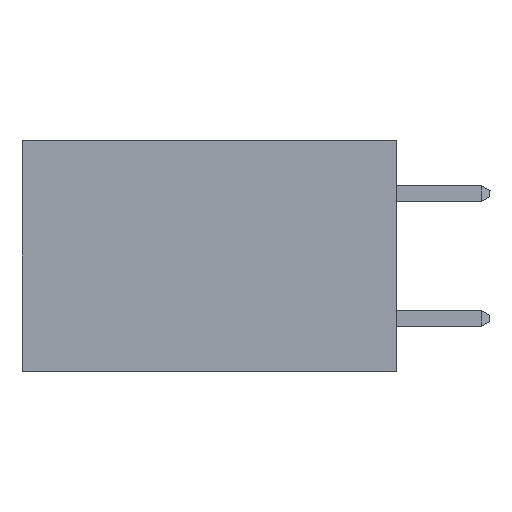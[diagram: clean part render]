
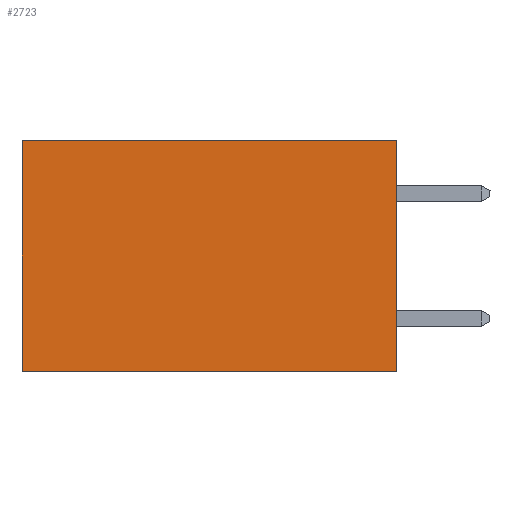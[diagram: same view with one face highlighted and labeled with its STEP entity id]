
A CAD part, left-side view. The second image highlights one B-rep face of the part: STEP entity #2723.
In plain terms, the highlighted planar face has unit normal (-1, 0, 0).
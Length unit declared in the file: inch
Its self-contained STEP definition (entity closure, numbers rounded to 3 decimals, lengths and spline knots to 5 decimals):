
#710 = VERTEX_POINT ( 'NONE', #7109 ) ;
#1138 = LINE ( 'NONE', #8458, #4950 ) ;
#1165 = CARTESIAN_POINT ( 'NONE',  ( 0.298, 0., 0. ) ) ;
#1316 = DIRECTION ( 'NONE',  ( 0., 0., -1. ) ) ;
#2104 = CARTESIAN_POINT ( 'NONE',  ( 0.298, 0., 0. ) ) ;
#2223 = VERTEX_POINT ( 'NONE', #3857 ) ;
#2297 = CARTESIAN_POINT ( 'NONE',  ( 0.298, 0., -0.37 ) ) ;
#2399 = ORIENTED_EDGE ( 'NONE', *, *, #8453, .T. ) ;
#2422 = DIRECTION ( 'NONE',  ( 0., 1., 0. ) ) ;
#2493 = DIRECTION ( 'NONE',  ( 0., 1., 0. ) ) ;
#2633 = ORIENTED_EDGE ( 'NONE', *, *, #3629, .F. ) ;
#2723 = ADVANCED_FACE ( 'NONE', ( #4390 ), #8285, .F. ) ;
#3629 = EDGE_CURVE ( 'NONE', #710, #7386, #8095, .T. ) ;
#3857 = CARTESIAN_POINT ( 'NONE',  ( 0.298, 0., 0. ) ) ;
#3867 = VECTOR ( 'NONE', #2422, 39.37008 ) ;
#4100 = ORIENTED_EDGE ( 'NONE', *, *, #7419, .F. ) ;
#4301 = CARTESIAN_POINT ( 'NONE',  ( 0.298, 0.6, 0. ) ) ;
#4390 = FACE_OUTER_BOUND ( 'NONE', #7220, .T. ) ;
#4600 = LINE ( 'NONE', #2104, #6430 ) ;
#4950 = VECTOR ( 'NONE', #6303, 39.37008 ) ;
#4968 = DIRECTION ( 'NONE',  ( 0., 0., -1. ) ) ;
#5902 = LINE ( 'NONE', #6170, #3867 ) ;
#6170 = CARTESIAN_POINT ( 'NONE',  ( 0.298, 0., 0. ) ) ;
#6303 = DIRECTION ( 'NONE',  ( 0., 0., -1. ) ) ;
#6430 = VECTOR ( 'NONE', #1316, 39.37008 ) ;
#6781 = ORIENTED_EDGE ( 'NONE', *, *, #9575, .T. ) ;
#6964 = DIRECTION ( 'NONE',  ( 1., 0., 0. ) ) ;
#7109 = CARTESIAN_POINT ( 'NONE',  ( 0.298, 0., -0.37 ) ) ;
#7220 = EDGE_LOOP ( 'NONE', ( #2399, #2633, #4100, #6781 ) ) ;
#7386 = VERTEX_POINT ( 'NONE', #8014 ) ;
#7419 = EDGE_CURVE ( 'NONE', #2223, #710, #4600, .T. ) ;
#7643 = VECTOR ( 'NONE', #2493, 39.37008 ) ;
#8014 = CARTESIAN_POINT ( 'NONE',  ( 0.298, 0.6, -0.37 ) ) ;
#8095 = LINE ( 'NONE', #2297, #7643 ) ;
#8285 = PLANE ( 'NONE',  #9706 ) ;
#8453 = EDGE_CURVE ( 'NONE', #9197, #7386, #1138, .T. ) ;
#8458 = CARTESIAN_POINT ( 'NONE',  ( 0.298, 0.6, 0. ) ) ;
#9197 = VERTEX_POINT ( 'NONE', #4301 ) ;
#9575 = EDGE_CURVE ( 'NONE', #2223, #9197, #5902, .T. ) ;
#9706 = AXIS2_PLACEMENT_3D ( 'NONE', #1165, #6964, #4968 ) ;
